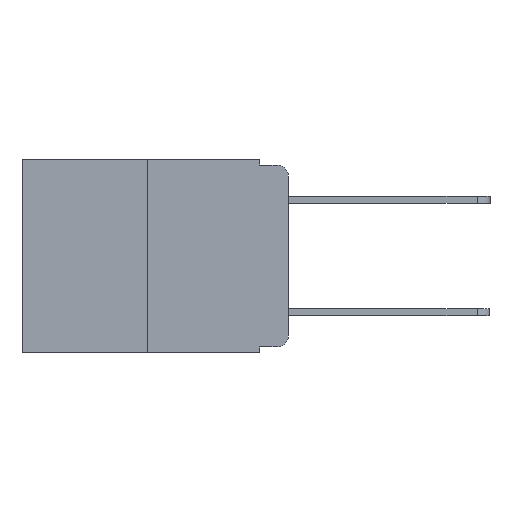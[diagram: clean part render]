
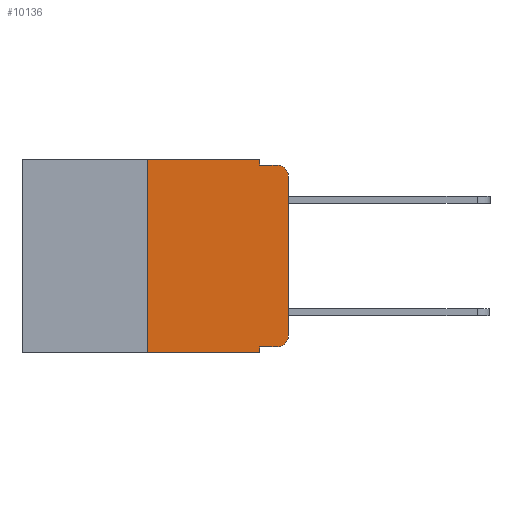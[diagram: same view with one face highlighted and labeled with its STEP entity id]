
A CAD part, left-side view. The second image highlights one B-rep face of the part: STEP entity #10136.
In plain terms, the highlighted planar face has unit normal (-1, 0, 0).
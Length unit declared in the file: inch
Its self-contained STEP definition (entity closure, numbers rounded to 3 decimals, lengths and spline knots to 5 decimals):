
#204 = CIRCLE ( 'NONE', #10817, 0.02 ) ;
#386 = ORIENTED_EDGE ( 'NONE', *, *, #2515, .T. ) ;
#880 = VERTEX_POINT ( 'NONE', #11297 ) ;
#985 = AXIS2_PLACEMENT_3D ( 'NONE', #14942, #6576, #16368 ) ;
#1314 = LINE ( 'NONE', #1423, #12053 ) ;
#1423 = CARTESIAN_POINT ( 'NONE',  ( 0., 0.051, 0. ) ) ;
#1683 = CARTESIAN_POINT ( 'NONE',  ( 0., 0.02, -0.333 ) ) ;
#1744 = LINE ( 'NONE', #1985, #12482 ) ;
#1807 = CARTESIAN_POINT ( 'NONE',  ( 0., 0., -0.313 ) ) ;
#1985 = CARTESIAN_POINT ( 'NONE',  ( 0., 0., 0. ) ) ;
#2263 = DIRECTION ( 'NONE',  ( 0., -1., 0. ) ) ;
#2515 = EDGE_CURVE ( 'NONE', #3920, #880, #1744, .T. ) ;
#2543 = LINE ( 'NONE', #7880, #9535 ) ;
#2594 = EDGE_CURVE ( 'NONE', #5285, #8364, #15764, .T. ) ;
#3104 = VERTEX_POINT ( 'NONE', #10040 ) ;
#3552 = EDGE_CURVE ( 'NONE', #3104, #7002, #15098, .T. ) ;
#3553 = EDGE_CURVE ( 'NONE', #8364, #3920, #204, .T. ) ;
#3678 = CARTESIAN_POINT ( 'NONE',  ( 0., 0.051, -0.01 ) ) ;
#3880 = DIRECTION ( 'NONE',  ( 0., 0., -1. ) ) ;
#3895 = VECTOR ( 'NONE', #5077, 39.37008 ) ;
#3920 = VERTEX_POINT ( 'NONE', #1807 ) ;
#4403 = VECTOR ( 'NONE', #4970, 39.37008 ) ;
#4970 = DIRECTION ( 'NONE',  ( 0., -1., 0. ) ) ;
#4973 = CARTESIAN_POINT ( 'NONE',  ( 0., 0.473, 0. ) ) ;
#5021 = CARTESIAN_POINT ( 'NONE',  ( 0., 0.051, -0.01 ) ) ;
#5077 = DIRECTION ( 'NONE',  ( 0., -1., 0. ) ) ;
#5261 = CARTESIAN_POINT ( 'NONE',  ( 0., 0.051, -0.343 ) ) ;
#5285 = VERTEX_POINT ( 'NONE', #6419 ) ;
#5294 = DIRECTION ( 'NONE',  ( 0., -1., 0. ) ) ;
#5795 = VECTOR ( 'NONE', #13057, 39.37008 ) ;
#6094 = ORIENTED_EDGE ( 'NONE', *, *, #12613, .T. ) ;
#6419 = CARTESIAN_POINT ( 'NONE',  ( 0., 0.051, -0.333 ) ) ;
#6576 = DIRECTION ( 'NONE',  ( 1., 0., 0. ) ) ;
#6838 = CARTESIAN_POINT ( 'NONE',  ( 0., 0.02, -0.01 ) ) ;
#7002 = VERTEX_POINT ( 'NONE', #16558 ) ;
#7634 = EDGE_CURVE ( 'NONE', #880, #18099, #14927, .T. ) ;
#7684 = CARTESIAN_POINT ( 'NONE',  ( 0., 0.25, -0.343 ) ) ;
#7874 = VECTOR ( 'NONE', #5294, 39.37008 ) ;
#7880 = CARTESIAN_POINT ( 'NONE',  ( 0., 0.473, -0.343 ) ) ;
#8171 = DIRECTION ( 'NONE',  ( 0., 0., -1. ) ) ;
#8187 = DIRECTION ( 'NONE',  ( -1., 0., 0. ) ) ;
#8190 = CARTESIAN_POINT ( 'NONE',  ( 0., 0.02, -0.313 ) ) ;
#8256 = CARTESIAN_POINT ( 'NONE',  ( 0., 0.02, -0.03 ) ) ;
#8364 = VERTEX_POINT ( 'NONE', #1683 ) ;
#8582 = AXIS2_PLACEMENT_3D ( 'NONE', #8256, #18067, #9663 ) ;
#8937 = EDGE_CURVE ( 'NONE', #7002, #17862, #1314, .T. ) ;
#9110 = ORIENTED_EDGE ( 'NONE', *, *, #7634, .T. ) ;
#9431 = ORIENTED_EDGE ( 'NONE', *, *, #3553, .T. ) ;
#9535 = VECTOR ( 'NONE', #2263, 39.37008 ) ;
#9593 = FACE_OUTER_BOUND ( 'NONE', #15462, .T. ) ;
#9663 = DIRECTION ( 'NONE',  ( 0., 0., -1. ) ) ;
#9942 = LINE ( 'NONE', #11648, #5795 ) ;
#10040 = CARTESIAN_POINT ( 'NONE',  ( 0., 0.25, 0. ) ) ;
#10136 = ADVANCED_FACE ( 'NONE', ( #9593 ), #13539, .F. ) ;
#10817 = AXIS2_PLACEMENT_3D ( 'NONE', #8190, #8187, #8171 ) ;
#11297 = CARTESIAN_POINT ( 'NONE',  ( 0., 0., -0.03 ) ) ;
#11382 = CARTESIAN_POINT ( 'NONE',  ( 0., 0.051, -0.333 ) ) ;
#11648 = CARTESIAN_POINT ( 'NONE',  ( 0., 0.25, 0. ) ) ;
#12053 = VECTOR ( 'NONE', #14093, 39.37008 ) ;
#12482 = VECTOR ( 'NONE', #15428, 39.37008 ) ;
#12520 = VERTEX_POINT ( 'NONE', #7684 ) ;
#12613 = EDGE_CURVE ( 'NONE', #12520, #13095, #2543, .T. ) ;
#13057 = DIRECTION ( 'NONE',  ( 0., 0., 1. ) ) ;
#13095 = VERTEX_POINT ( 'NONE', #5261 ) ;
#13496 = EDGE_CURVE ( 'NONE', #12520, #3104, #9942, .T. ) ;
#13497 = ORIENTED_EDGE ( 'NONE', *, *, #8937, .F. ) ;
#13539 = PLANE ( 'NONE',  #985 ) ;
#14093 = DIRECTION ( 'NONE',  ( 0., 0., -1. ) ) ;
#14371 = ORIENTED_EDGE ( 'NONE', *, *, #14424, .F. ) ;
#14406 = VECTOR ( 'NONE', #3880, 39.37008 ) ;
#14413 = ORIENTED_EDGE ( 'NONE', *, *, #16099, .F. ) ;
#14424 = EDGE_CURVE ( 'NONE', #5285, #13095, #18160, .T. ) ;
#14927 = CIRCLE ( 'NONE', #8582, 0.02 ) ;
#14942 = CARTESIAN_POINT ( 'NONE',  ( 0., 0.473, 0. ) ) ;
#15034 = LINE ( 'NONE', #3678, #3895 ) ;
#15088 = ORIENTED_EDGE ( 'NONE', *, *, #13496, .F. ) ;
#15098 = LINE ( 'NONE', #4973, #4403 ) ;
#15355 = ORIENTED_EDGE ( 'NONE', *, *, #2594, .T. ) ;
#15428 = DIRECTION ( 'NONE',  ( 0., 0., 1. ) ) ;
#15462 = EDGE_LOOP ( 'NONE', ( #386, #9110, #14413, #13497, #17180, #15088, #6094, #14371, #15355, #9431 ) ) ;
#15764 = LINE ( 'NONE', #11382, #7874 ) ;
#16099 = EDGE_CURVE ( 'NONE', #17862, #18099, #15034, .T. ) ;
#16368 = DIRECTION ( 'NONE',  ( 0., 0., -1. ) ) ;
#16477 = CARTESIAN_POINT ( 'NONE',  ( 0., 0.051, 0. ) ) ;
#16558 = CARTESIAN_POINT ( 'NONE',  ( 0., 0.051, 0. ) ) ;
#17180 = ORIENTED_EDGE ( 'NONE', *, *, #3552, .F. ) ;
#17862 = VERTEX_POINT ( 'NONE', #5021 ) ;
#18067 = DIRECTION ( 'NONE',  ( -1., 0., 0. ) ) ;
#18099 = VERTEX_POINT ( 'NONE', #6838 ) ;
#18160 = LINE ( 'NONE', #16477, #14406 ) ;
